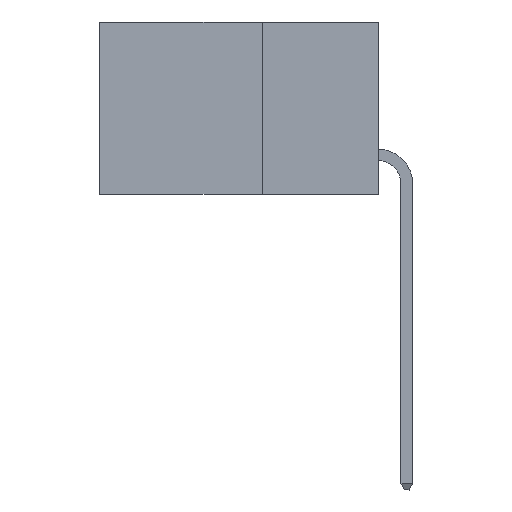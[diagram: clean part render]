
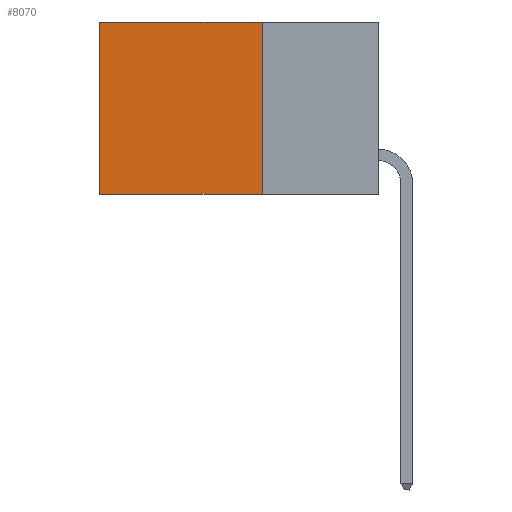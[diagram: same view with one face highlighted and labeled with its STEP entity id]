
A CAD part, left-side view. The second image highlights one B-rep face of the part: STEP entity #8070.
In plain terms, the highlighted planar face has unit normal (-1, 0, 0).
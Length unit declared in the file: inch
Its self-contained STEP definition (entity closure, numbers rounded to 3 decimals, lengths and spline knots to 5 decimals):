
#59 = CARTESIAN_POINT ( 'NONE',  ( 0.2615, 0.6, -0.37 ) ) ;
#806 = VERTEX_POINT ( 'NONE', #8762 ) ;
#2226 = CARTESIAN_POINT ( 'NONE',  ( 0.2615, 0.25, 0. ) ) ;
#2286 = CARTESIAN_POINT ( 'NONE',  ( 0.2615, 0.25, -0.37 ) ) ;
#2881 = CARTESIAN_POINT ( 'NONE',  ( 0.2615, 0.25, 0. ) ) ;
#2974 = DIRECTION ( 'NONE',  ( 0., 1., 0. ) ) ;
#3586 = PLANE ( 'NONE',  #13115 ) ;
#3721 = LINE ( 'NONE', #17961, #13207 ) ;
#4077 = EDGE_CURVE ( 'NONE', #15571, #4470, #10033, .T. ) ;
#4470 = VERTEX_POINT ( 'NONE', #12810 ) ;
#6067 = EDGE_CURVE ( 'NONE', #4470, #10240, #18053, .T. ) ;
#6269 = VECTOR ( 'NONE', #2974, 39.37008 ) ;
#6285 = FACE_OUTER_BOUND ( 'NONE', #7066, .T. ) ;
#6430 = VECTOR ( 'NONE', #10073, 39.37008 ) ;
#6509 = DIRECTION ( 'NONE',  ( 0., 0., -1. ) ) ;
#7066 = EDGE_LOOP ( 'NONE', ( #16472, #17668, #17581, #17260 ) ) ;
#7956 = DIRECTION ( 'NONE',  ( 1., 0., 0. ) ) ;
#8070 = ADVANCED_FACE ( 'NONE', ( #6285 ), #3586, .F. ) ;
#8762 = CARTESIAN_POINT ( 'NONE',  ( 0.2615, 0.25, -0.37 ) ) ;
#9516 = VECTOR ( 'NONE', #16503, 39.37008 ) ;
#9720 = EDGE_CURVE ( 'NONE', #15571, #806, #3721, .T. ) ;
#10033 = LINE ( 'NONE', #2881, #6269 ) ;
#10073 = DIRECTION ( 'NONE',  ( 0., 1., 0. ) ) ;
#10166 = CARTESIAN_POINT ( 'NONE',  ( 0.2615, 0.25, -0.37 ) ) ;
#10240 = VERTEX_POINT ( 'NONE', #59 ) ;
#10838 = EDGE_CURVE ( 'NONE', #806, #10240, #12921, .T. ) ;
#12810 = CARTESIAN_POINT ( 'NONE',  ( 0.2615, 0.6, 0. ) ) ;
#12921 = LINE ( 'NONE', #10166, #6430 ) ;
#13115 = AXIS2_PLACEMENT_3D ( 'NONE', #2286, #7956, #13598 ) ;
#13207 = VECTOR ( 'NONE', #6509, 39.37008 ) ;
#13598 = DIRECTION ( 'NONE',  ( 0., 0., -1. ) ) ;
#15571 = VERTEX_POINT ( 'NONE', #2226 ) ;
#16472 = ORIENTED_EDGE ( 'NONE', *, *, #6067, .T. ) ;
#16503 = DIRECTION ( 'NONE',  ( 0., 0., -1. ) ) ;
#16858 = CARTESIAN_POINT ( 'NONE',  ( 0.2615, 0.6, -0.37 ) ) ;
#17260 = ORIENTED_EDGE ( 'NONE', *, *, #4077, .T. ) ;
#17581 = ORIENTED_EDGE ( 'NONE', *, *, #9720, .F. ) ;
#17668 = ORIENTED_EDGE ( 'NONE', *, *, #10838, .F. ) ;
#17961 = CARTESIAN_POINT ( 'NONE',  ( 0.2615, 0.25, -0.37 ) ) ;
#18053 = LINE ( 'NONE', #16858, #9516 ) ;
